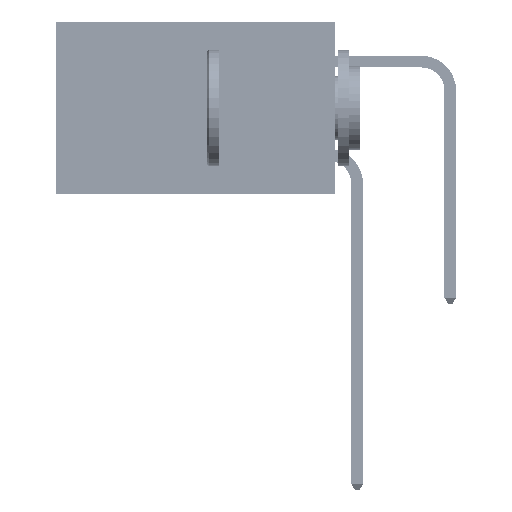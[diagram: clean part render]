
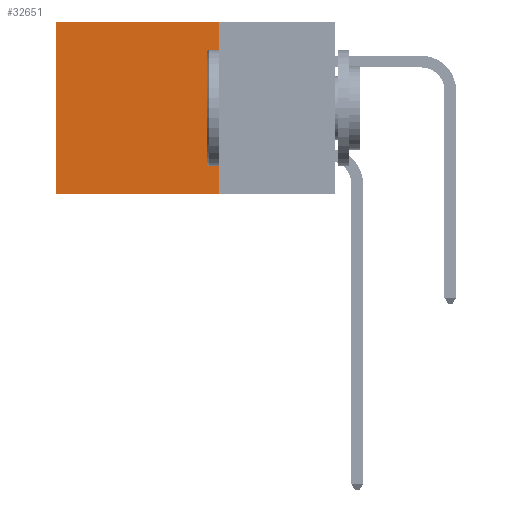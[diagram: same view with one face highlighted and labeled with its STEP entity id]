
A CAD part, left-side view. The second image highlights one B-rep face of the part: STEP entity #32651.
In plain terms, the highlighted planar face has unit normal (-1, 0, 0).
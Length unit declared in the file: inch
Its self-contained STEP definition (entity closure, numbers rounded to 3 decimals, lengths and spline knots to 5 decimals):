
#2950 = LINE ( 'NONE', #20744, #25967 ) ;
#6892 = LINE ( 'NONE', #22062, #21241 ) ;
#11396 = DIRECTION ( 'NONE',  ( 0., 1., 0. ) ) ;
#11731 = DIRECTION ( 'NONE',  ( 1., 0., 0. ) ) ;
#12311 = VERTEX_POINT ( 'NONE', #45718 ) ;
#12852 = VECTOR ( 'NONE', #11396, 39.37008 ) ;
#13389 = DIRECTION ( 'NONE',  ( 0., 0., -1. ) ) ;
#13889 = CARTESIAN_POINT ( 'NONE',  ( 0.2875, 0.6, 0. ) ) ;
#16590 = VERTEX_POINT ( 'NONE', #21327 ) ;
#16647 = ORIENTED_EDGE ( 'NONE', *, *, #20765, .T. ) ;
#17974 = AXIS2_PLACEMENT_3D ( 'NONE', #25544, #11731, #33561 ) ;
#19077 = CARTESIAN_POINT ( 'NONE',  ( 0.2875, 0.25, -0.37 ) ) ;
#20024 = ORIENTED_EDGE ( 'NONE', *, *, #42170, .T. ) ;
#20256 = DIRECTION ( 'NONE',  ( 0., 1., 0. ) ) ;
#20744 = CARTESIAN_POINT ( 'NONE',  ( 0.2875, 0.6, 0. ) ) ;
#20765 = EDGE_CURVE ( 'NONE', #34370, #16590, #2950, .T. ) ;
#21241 = VECTOR ( 'NONE', #22547, 39.37008 ) ;
#21327 = CARTESIAN_POINT ( 'NONE',  ( 0.2875, 0.6, -0.37 ) ) ;
#22062 = CARTESIAN_POINT ( 'NONE',  ( 0.2875, 0.25, 0. ) ) ;
#22547 = DIRECTION ( 'NONE',  ( 0., 0., -1. ) ) ;
#23882 = VECTOR ( 'NONE', #20256, 39.37008 ) ;
#25544 = CARTESIAN_POINT ( 'NONE',  ( 0.2875, 0.25, 0. ) ) ;
#25602 = VERTEX_POINT ( 'NONE', #44117 ) ;
#25967 = VECTOR ( 'NONE', #13389, 39.37008 ) ;
#28942 = LINE ( 'NONE', #19077, #12852 ) ;
#30915 = EDGE_CURVE ( 'NONE', #12311, #16590, #28942, .T. ) ;
#32651 = ADVANCED_FACE ( 'NONE', ( #32798 ), #47587, .F. ) ;
#32798 = FACE_OUTER_BOUND ( 'NONE', #40242, .T. ) ;
#33561 = DIRECTION ( 'NONE',  ( 0., 0., -1. ) ) ;
#34370 = VERTEX_POINT ( 'NONE', #13889 ) ;
#38249 = CARTESIAN_POINT ( 'NONE',  ( 0.2875, 0.25, 0. ) ) ;
#40242 = EDGE_LOOP ( 'NONE', ( #16647, #44684, #41069, #20024 ) ) ;
#41069 = ORIENTED_EDGE ( 'NONE', *, *, #43467, .F. ) ;
#42170 = EDGE_CURVE ( 'NONE', #25602, #34370, #43446, .T. ) ;
#43446 = LINE ( 'NONE', #38249, #23882 ) ;
#43467 = EDGE_CURVE ( 'NONE', #25602, #12311, #6892, .T. ) ;
#44117 = CARTESIAN_POINT ( 'NONE',  ( 0.2875, 0.25, 0. ) ) ;
#44684 = ORIENTED_EDGE ( 'NONE', *, *, #30915, .F. ) ;
#45718 = CARTESIAN_POINT ( 'NONE',  ( 0.2875, 0.25, -0.37 ) ) ;
#47587 = PLANE ( 'NONE',  #17974 ) ;
